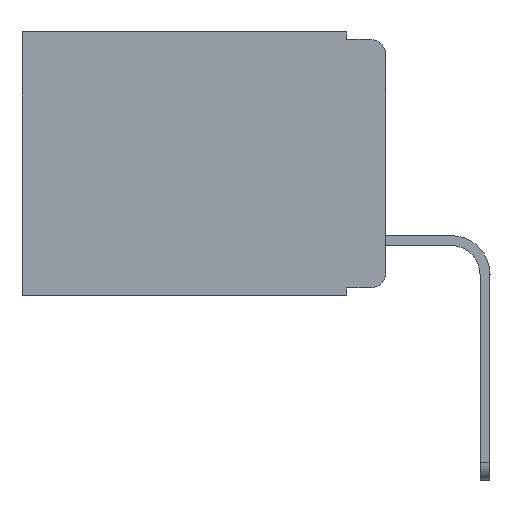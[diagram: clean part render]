
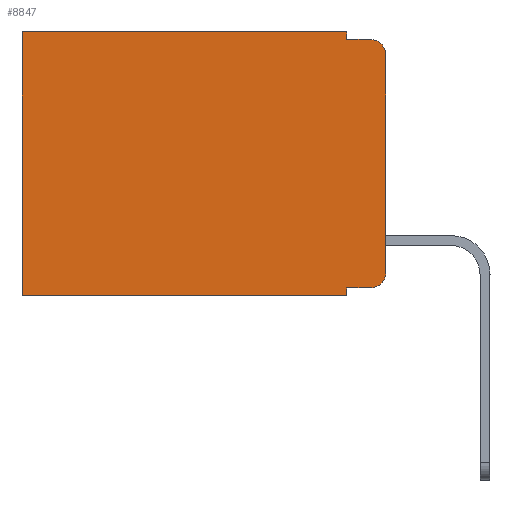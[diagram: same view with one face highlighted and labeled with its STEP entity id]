
A CAD part, left-side view. The second image highlights one B-rep face of the part: STEP entity #8847.
In plain terms, the highlighted planar face has unit normal (-1, 0, 0).
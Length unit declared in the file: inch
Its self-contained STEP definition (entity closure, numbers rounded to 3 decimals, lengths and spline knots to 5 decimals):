
#221 = EDGE_CURVE ( 'NONE', #11062, #2678, #5977, .T. ) ;
#293 = EDGE_CURVE ( 'NONE', #12968, #2657, #390, .T. ) ;
#390 = LINE ( 'NONE', #19495, #12736 ) ;
#461 = ORIENTED_EDGE ( 'NONE', *, *, #8019, .T. ) ;
#620 = VECTOR ( 'NONE', #11194, 39.37008 ) ;
#664 = LINE ( 'NONE', #2550, #923 ) ;
#738 = ORIENTED_EDGE ( 'NONE', *, *, #19038, .F. ) ;
#820 = ORIENTED_EDGE ( 'NONE', *, *, #16936, .T. ) ;
#923 = VECTOR ( 'NONE', #4028, 39.37008 ) ;
#1019 = CARTESIAN_POINT ( 'NONE',  ( 0.298, 0.02, -0.333 ) ) ;
#1089 = EDGE_CURVE ( 'NONE', #4261, #2678, #1666, .T. ) ;
#1264 = LINE ( 'NONE', #18381, #5264 ) ;
#1321 = CARTESIAN_POINT ( 'NONE',  ( 0.298, 0.02, -0.01 ) ) ;
#1466 = CARTESIAN_POINT ( 'NONE',  ( 0.298, 0., 0. ) ) ;
#1666 = LINE ( 'NONE', #14808, #620 ) ;
#1857 = AXIS2_PLACEMENT_3D ( 'NONE', #4212, #17558, #19418 ) ;
#1872 = LINE ( 'NONE', #9082, #5637 ) ;
#1968 = AXIS2_PLACEMENT_3D ( 'NONE', #13924, #2291, #3919 ) ;
#2162 = CARTESIAN_POINT ( 'NONE',  ( 0.298, 0., -0.313 ) ) ;
#2291 = DIRECTION ( 'NONE',  ( -1., 0., 0. ) ) ;
#2489 = CIRCLE ( 'NONE', #1857, 0.02 ) ;
#2550 = CARTESIAN_POINT ( 'NONE',  ( 0.298, 0.051, -0.333 ) ) ;
#2657 = VERTEX_POINT ( 'NONE', #9571 ) ;
#2678 = VERTEX_POINT ( 'NONE', #1321 ) ;
#3469 = CARTESIAN_POINT ( 'NONE',  ( 0.298, 0.051, 0. ) ) ;
#3550 = ORIENTED_EDGE ( 'NONE', *, *, #3968, .T. ) ;
#3710 = CARTESIAN_POINT ( 'NONE',  ( 0.298, 0.473, 0. ) ) ;
#3789 = CARTESIAN_POINT ( 'NONE',  ( 0.298, 0.051, -0.333 ) ) ;
#3919 = DIRECTION ( 'NONE',  ( 0., 0., -1. ) ) ;
#3968 = EDGE_CURVE ( 'NONE', #4325, #13085, #2489, .T. ) ;
#4028 = DIRECTION ( 'NONE',  ( 0., -1., 0. ) ) ;
#4212 = CARTESIAN_POINT ( 'NONE',  ( 0.298, 0.02, -0.313 ) ) ;
#4261 = VERTEX_POINT ( 'NONE', #7751 ) ;
#4325 = VERTEX_POINT ( 'NONE', #1019 ) ;
#4675 = VERTEX_POINT ( 'NONE', #3789 ) ;
#4925 = VERTEX_POINT ( 'NONE', #5116 ) ;
#5116 = CARTESIAN_POINT ( 'NONE',  ( 0.298, 0.051, 0. ) ) ;
#5264 = VECTOR ( 'NONE', #20313, 39.37008 ) ;
#5618 = VECTOR ( 'NONE', #18339, 39.37008 ) ;
#5637 = VECTOR ( 'NONE', #10746, 39.37008 ) ;
#5977 = CIRCLE ( 'NONE', #1968, 0.02 ) ;
#7121 = ORIENTED_EDGE ( 'NONE', *, *, #16681, .F. ) ;
#7424 = ORIENTED_EDGE ( 'NONE', *, *, #15163, .F. ) ;
#7751 = CARTESIAN_POINT ( 'NONE',  ( 0.298, 0.051, -0.01 ) ) ;
#8019 = EDGE_CURVE ( 'NONE', #4675, #4325, #664, .T. ) ;
#8027 = ORIENTED_EDGE ( 'NONE', *, *, #221, .T. ) ;
#8390 = EDGE_LOOP ( 'NONE', ( #7121, #8027, #11190, #7424, #820, #14066, #14937, #738, #461, #3550 ) ) ;
#8847 = ADVANCED_FACE ( 'NONE', ( #8917 ), #21614, .F. ) ;
#8917 = FACE_OUTER_BOUND ( 'NONE', #8390, .T. ) ;
#9082 = CARTESIAN_POINT ( 'NONE',  ( 0.298, 0., 0. ) ) ;
#9571 = CARTESIAN_POINT ( 'NONE',  ( 0.298, 0.473, -0.343 ) ) ;
#10137 = VERTEX_POINT ( 'NONE', #3710 ) ;
#10709 = CARTESIAN_POINT ( 'NONE',  ( 0.298, 0.473, 0. ) ) ;
#10746 = DIRECTION ( 'NONE',  ( 0., 0., -1. ) ) ;
#11062 = VERTEX_POINT ( 'NONE', #13478 ) ;
#11190 = ORIENTED_EDGE ( 'NONE', *, *, #1089, .F. ) ;
#11194 = DIRECTION ( 'NONE',  ( 0., -1., 0. ) ) ;
#12046 = AXIS2_PLACEMENT_3D ( 'NONE', #16676, #15046, #20095 ) ;
#12736 = VECTOR ( 'NONE', #19573, 39.37008 ) ;
#12926 = CARTESIAN_POINT ( 'NONE',  ( 0.298, 0.051, -0.343 ) ) ;
#12960 = VECTOR ( 'NONE', #18405, 39.37008 ) ;
#12968 = VERTEX_POINT ( 'NONE', #12926 ) ;
#13085 = VERTEX_POINT ( 'NONE', #2162 ) ;
#13478 = CARTESIAN_POINT ( 'NONE',  ( 0.298, 0., -0.03 ) ) ;
#13924 = CARTESIAN_POINT ( 'NONE',  ( 0.298, 0.02, -0.03 ) ) ;
#14066 = ORIENTED_EDGE ( 'NONE', *, *, #18643, .T. ) ;
#14698 = VECTOR ( 'NONE', #20802, 39.37008 ) ;
#14808 = CARTESIAN_POINT ( 'NONE',  ( 0.298, 0.051, -0.01 ) ) ;
#14937 = ORIENTED_EDGE ( 'NONE', *, *, #293, .F. ) ;
#15046 = DIRECTION ( 'NONE',  ( 1., 0., 0. ) ) ;
#15163 = EDGE_CURVE ( 'NONE', #4925, #4261, #21748, .T. ) ;
#15769 = LINE ( 'NONE', #10709, #14698 ) ;
#16676 = CARTESIAN_POINT ( 'NONE',  ( 0.298, 0., 0. ) ) ;
#16681 = EDGE_CURVE ( 'NONE', #11062, #13085, #1872, .T. ) ;
#16936 = EDGE_CURVE ( 'NONE', #4925, #10137, #17935, .T. ) ;
#17558 = DIRECTION ( 'NONE',  ( -1., 0., 0. ) ) ;
#17935 = LINE ( 'NONE', #1466, #5618 ) ;
#18339 = DIRECTION ( 'NONE',  ( 0., 1., 0. ) ) ;
#18381 = CARTESIAN_POINT ( 'NONE',  ( 0.298, 0.051, 0. ) ) ;
#18405 = DIRECTION ( 'NONE',  ( 0., 0., -1. ) ) ;
#18643 = EDGE_CURVE ( 'NONE', #10137, #2657, #15769, .T. ) ;
#19038 = EDGE_CURVE ( 'NONE', #4675, #12968, #1264, .T. ) ;
#19418 = DIRECTION ( 'NONE',  ( 0., 0., -1. ) ) ;
#19495 = CARTESIAN_POINT ( 'NONE',  ( 0.298, 0., -0.343 ) ) ;
#19573 = DIRECTION ( 'NONE',  ( 0., 1., 0. ) ) ;
#20095 = DIRECTION ( 'NONE',  ( 0., 0., -1. ) ) ;
#20313 = DIRECTION ( 'NONE',  ( 0., 0., -1. ) ) ;
#20802 = DIRECTION ( 'NONE',  ( 0., 0., -1. ) ) ;
#21614 = PLANE ( 'NONE',  #12046 ) ;
#21748 = LINE ( 'NONE', #3469, #12960 ) ;
